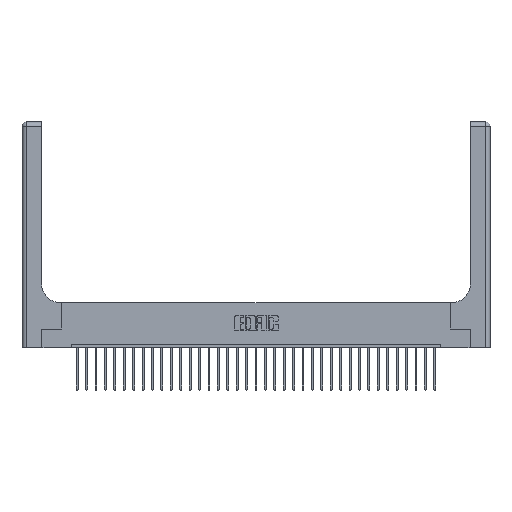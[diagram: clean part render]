
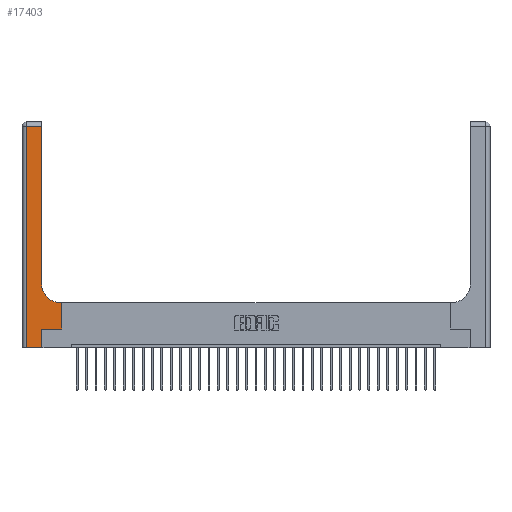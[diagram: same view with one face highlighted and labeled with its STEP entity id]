
A CAD part, top view. The second image highlights one B-rep face of the part: STEP entity #17403.
In plain terms, the highlighted planar face has unit normal (0, 0, 1).
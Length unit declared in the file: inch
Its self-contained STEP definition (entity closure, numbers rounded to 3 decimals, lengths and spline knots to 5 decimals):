
#298 = DIRECTION ( 'NONE',  ( 1., 0., 0. ) ) ;
#1067 = DIRECTION ( 'NONE',  ( -1., 0., 0. ) ) ;
#1548 = EDGE_CURVE ( 'NONE', #18386, #29766, #21369, .T. ) ;
#1754 = CARTESIAN_POINT ( 'NONE',  ( 0.528, 0.25, 0.37 ) ) ;
#3658 = CARTESIAN_POINT ( 'NONE',  ( 0.06, 3., 0.37 ) ) ;
#3934 = ORIENTED_EDGE ( 'NONE', *, *, #5228, .T. ) ;
#4122 = DIRECTION ( 'NONE',  ( 0., -1., 0. ) ) ;
#4472 = AXIS2_PLACEMENT_3D ( 'NONE', #15534, #20093, #13663 ) ;
#4832 = DIRECTION ( 'NONE',  ( 0., 1., 0. ) ) ;
#5041 = VERTEX_POINT ( 'NONE', #9068 ) ;
#5193 = VECTOR ( 'NONE', #17105, 39.37008 ) ;
#5228 = EDGE_CURVE ( 'NONE', #15947, #8114, #15754, .T. ) ;
#5731 = VERTEX_POINT ( 'NONE', #17926 ) ;
#5805 = FACE_OUTER_BOUND ( 'NONE', #19539, .T. ) ;
#5812 = CARTESIAN_POINT ( 'NONE',  ( 0.06, 0., 0.37 ) ) ;
#6031 = VECTOR ( 'NONE', #7115, 39.37008 ) ;
#6999 = ORIENTED_EDGE ( 'NONE', *, *, #28507, .T. ) ;
#7037 = ORIENTED_EDGE ( 'NONE', *, *, #1548, .T. ) ;
#7048 = CARTESIAN_POINT ( 'NONE',  ( 0.06, 2.94, 0.37 ) ) ;
#7115 = DIRECTION ( 'NONE',  ( 1., 0., 0. ) ) ;
#7786 = CARTESIAN_POINT ( 'NONE',  ( 0.26, 0.6, 0.37 ) ) ;
#7835 = CARTESIAN_POINT ( 'NONE',  ( 0.528, 0.6, 0.37 ) ) ;
#7927 = CIRCLE ( 'NONE', #4472, 0.25 ) ;
#8114 = VERTEX_POINT ( 'NONE', #5812 ) ;
#8458 = CARTESIAN_POINT ( 'NONE',  ( 0., 3., 0.37 ) ) ;
#8793 = DIRECTION ( 'NONE',  ( 0., 1., 0. ) ) ;
#8915 = ORIENTED_EDGE ( 'NONE', *, *, #28469, .T. ) ;
#9068 = CARTESIAN_POINT ( 'NONE',  ( 0.265, 0., 0.37 ) ) ;
#9450 = CARTESIAN_POINT ( 'NONE',  ( 0.265, 0.25, 0.37 ) ) ;
#10725 = PLANE ( 'NONE',  #18071 ) ;
#11066 = CARTESIAN_POINT ( 'NONE',  ( 0.26, 3., 0.37 ) ) ;
#11430 = CARTESIAN_POINT ( 'NONE',  ( 0.51, 0.6, 0.37 ) ) ;
#11540 = CARTESIAN_POINT ( 'NONE',  ( 0.26, 2.94, 0.37 ) ) ;
#11625 = EDGE_CURVE ( 'NONE', #8114, #5041, #12262, .T. ) ;
#12262 = LINE ( 'NONE', #19148, #28964 ) ;
#12397 = ORIENTED_EDGE ( 'NONE', *, *, #15872, .T. ) ;
#13663 = DIRECTION ( 'NONE',  ( 1., 0., 0. ) ) ;
#14208 = CARTESIAN_POINT ( 'NONE',  ( 0., 2.94, 0.37 ) ) ;
#14681 = LINE ( 'NONE', #7786, #5193 ) ;
#15454 = VECTOR ( 'NONE', #18078, 39.37008 ) ;
#15534 = CARTESIAN_POINT ( 'NONE',  ( 0.51, 0.85, 0.37 ) ) ;
#15754 = LINE ( 'NONE', #3658, #29207 ) ;
#15872 = EDGE_CURVE ( 'NONE', #5041, #5731, #20847, .T. ) ;
#15947 = VERTEX_POINT ( 'NONE', #7048 ) ;
#16182 = ORIENTED_EDGE ( 'NONE', *, *, #25217, .T. ) ;
#16655 = VERTEX_POINT ( 'NONE', #11540 ) ;
#17069 = CARTESIAN_POINT ( 'NONE',  ( 0.26, 0.85, 0.37 ) ) ;
#17105 = DIRECTION ( 'NONE',  ( -1., 0., 0. ) ) ;
#17337 = VECTOR ( 'NONE', #4832, 39.37008 ) ;
#17403 = ADVANCED_FACE ( 'NONE', ( #5805 ), #10725, .F. ) ;
#17926 = CARTESIAN_POINT ( 'NONE',  ( 0.265, 0.25, 0.37 ) ) ;
#18038 = VERTEX_POINT ( 'NONE', #11430 ) ;
#18071 = AXIS2_PLACEMENT_3D ( 'NONE', #8458, #24809, #1067 ) ;
#18078 = DIRECTION ( 'NONE',  ( 0., 1., 0. ) ) ;
#18386 = VERTEX_POINT ( 'NONE', #1754 ) ;
#19148 = CARTESIAN_POINT ( 'NONE',  ( 0., 0., 0.37 ) ) ;
#19539 = EDGE_LOOP ( 'NONE', ( #6999, #8915, #3934, #27131, #12397, #22710, #7037, #26307, #16182 ) ) ;
#20093 = DIRECTION ( 'NONE',  ( 0., 0., -1. ) ) ;
#20847 = LINE ( 'NONE', #30147, #15454 ) ;
#21219 = CARTESIAN_POINT ( 'NONE',  ( 0.528, 0.25, 0.37 ) ) ;
#21262 = DIRECTION ( 'NONE',  ( -1., 0., 0. ) ) ;
#21369 = LINE ( 'NONE', #21219, #17337 ) ;
#22710 = ORIENTED_EDGE ( 'NONE', *, *, #27632, .T. ) ;
#23771 = VECTOR ( 'NONE', #8793, 39.37008 ) ;
#24809 = DIRECTION ( 'NONE',  ( 0., 0., -1. ) ) ;
#24990 = LINE ( 'NONE', #11066, #23771 ) ;
#25217 = EDGE_CURVE ( 'NONE', #18038, #27780, #7927, .T. ) ;
#25353 = LINE ( 'NONE', #9450, #6031 ) ;
#26307 = ORIENTED_EDGE ( 'NONE', *, *, #28682, .T. ) ;
#27131 = ORIENTED_EDGE ( 'NONE', *, *, #11625, .T. ) ;
#27399 = LINE ( 'NONE', #14208, #29609 ) ;
#27632 = EDGE_CURVE ( 'NONE', #5731, #18386, #25353, .T. ) ;
#27780 = VERTEX_POINT ( 'NONE', #17069 ) ;
#28469 = EDGE_CURVE ( 'NONE', #16655, #15947, #27399, .T. ) ;
#28507 = EDGE_CURVE ( 'NONE', #27780, #16655, #24990, .T. ) ;
#28682 = EDGE_CURVE ( 'NONE', #29766, #18038, #14681, .T. ) ;
#28964 = VECTOR ( 'NONE', #298, 39.37008 ) ;
#29207 = VECTOR ( 'NONE', #4122, 39.37008 ) ;
#29609 = VECTOR ( 'NONE', #21262, 39.37008 ) ;
#29766 = VERTEX_POINT ( 'NONE', #7835 ) ;
#30147 = CARTESIAN_POINT ( 'NONE',  ( 0.265, 0., 0.37 ) ) ;
